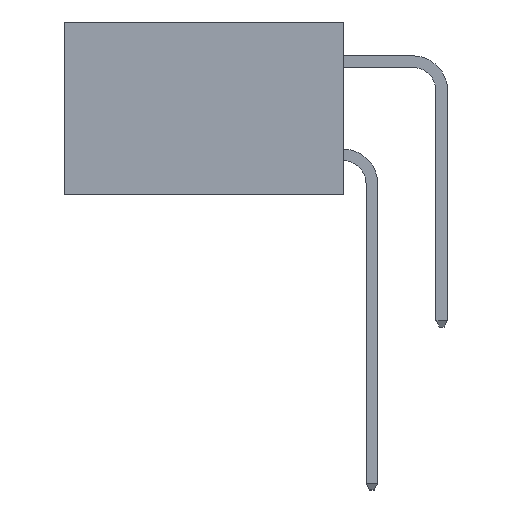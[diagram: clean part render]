
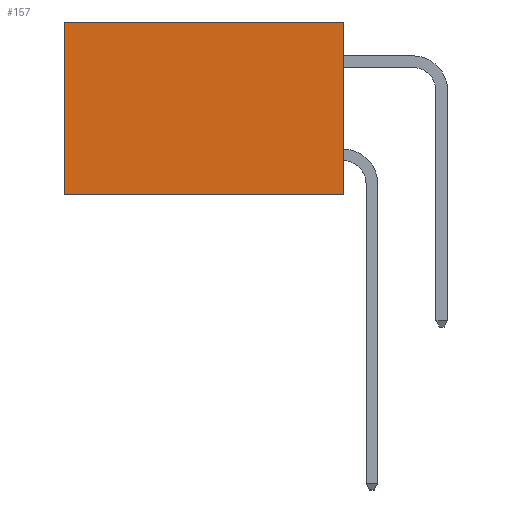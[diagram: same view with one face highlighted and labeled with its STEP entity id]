
A CAD part, left-side view. The second image highlights one B-rep face of the part: STEP entity #157.
In plain terms, the highlighted planar face has unit normal (-1, 0, 0).
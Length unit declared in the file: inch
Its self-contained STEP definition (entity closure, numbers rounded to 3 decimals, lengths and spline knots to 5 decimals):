
#157 = ADVANCED_FACE ( 'NONE', ( #3345 ), #8088, .F. ) ;
#681 = CARTESIAN_POINT ( 'NONE',  ( 0.2615, 0., -0.37 ) ) ;
#769 = ORIENTED_EDGE ( 'NONE', *, *, #9061, .T. ) ;
#778 = VERTEX_POINT ( 'NONE', #8372 ) ;
#1228 = ORIENTED_EDGE ( 'NONE', *, *, #12592, .F. ) ;
#1450 = DIRECTION ( 'NONE',  ( 1., 0., 0. ) ) ;
#1582 = DIRECTION ( 'NONE',  ( 0., 1., 0. ) ) ;
#1855 = EDGE_LOOP ( 'NONE', ( #769, #1228, #2614, #3628 ) ) ;
#2516 = CARTESIAN_POINT ( 'NONE',  ( 0.2615, 0.6, -0.37 ) ) ;
#2614 = ORIENTED_EDGE ( 'NONE', *, *, #7536, .F. ) ;
#2923 = LINE ( 'NONE', #8110, #8887 ) ;
#3345 = FACE_OUTER_BOUND ( 'NONE', #1855, .T. ) ;
#3628 = ORIENTED_EDGE ( 'NONE', *, *, #14123, .T. ) ;
#4890 = CARTESIAN_POINT ( 'NONE',  ( 0.2615, 0., 0. ) ) ;
#5381 = AXIS2_PLACEMENT_3D ( 'NONE', #681, #1450, #8893 ) ;
#5962 = LINE ( 'NONE', #6030, #11550 ) ;
#6030 = CARTESIAN_POINT ( 'NONE',  ( 0.2615, 0., -0.37 ) ) ;
#6067 = CARTESIAN_POINT ( 'NONE',  ( 0.2615, 0., -0.37 ) ) ;
#6332 = DIRECTION ( 'NONE',  ( 0., 0., -1. ) ) ;
#6337 = VERTEX_POINT ( 'NONE', #7111 ) ;
#7111 = CARTESIAN_POINT ( 'NONE',  ( 0.2615, 0., -0.37 ) ) ;
#7536 = EDGE_CURVE ( 'NONE', #9542, #6337, #13497, .T. ) ;
#8088 = PLANE ( 'NONE',  #5381 ) ;
#8110 = CARTESIAN_POINT ( 'NONE',  ( 0.2615, 0.6, -0.37 ) ) ;
#8301 = LINE ( 'NONE', #4890, #10910 ) ;
#8372 = CARTESIAN_POINT ( 'NONE',  ( 0.2615, 0.6, 0. ) ) ;
#8887 = VECTOR ( 'NONE', #12576, 39.37008 ) ;
#8893 = DIRECTION ( 'NONE',  ( 0., 0., -1. ) ) ;
#8957 = VERTEX_POINT ( 'NONE', #2516 ) ;
#9061 = EDGE_CURVE ( 'NONE', #778, #8957, #2923, .T. ) ;
#9542 = VERTEX_POINT ( 'NONE', #13872 ) ;
#10493 = VECTOR ( 'NONE', #6332, 39.37008 ) ;
#10910 = VECTOR ( 'NONE', #12615, 39.37008 ) ;
#11550 = VECTOR ( 'NONE', #1582, 39.37008 ) ;
#12576 = DIRECTION ( 'NONE',  ( 0., 0., -1. ) ) ;
#12592 = EDGE_CURVE ( 'NONE', #6337, #8957, #5962, .T. ) ;
#12615 = DIRECTION ( 'NONE',  ( 0., 1., 0. ) ) ;
#13497 = LINE ( 'NONE', #6067, #10493 ) ;
#13872 = CARTESIAN_POINT ( 'NONE',  ( 0.2615, 0., 0. ) ) ;
#14123 = EDGE_CURVE ( 'NONE', #9542, #778, #8301, .T. ) ;
